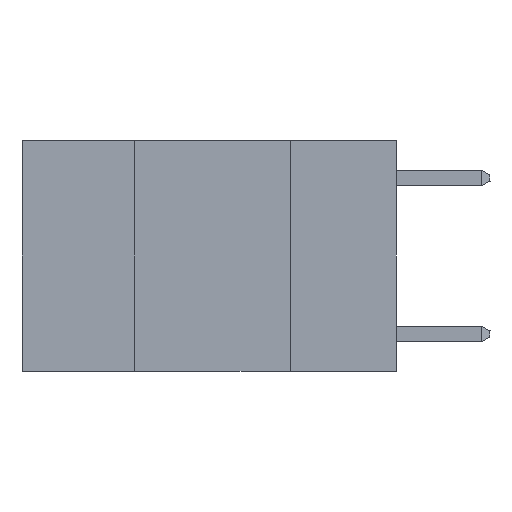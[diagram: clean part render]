
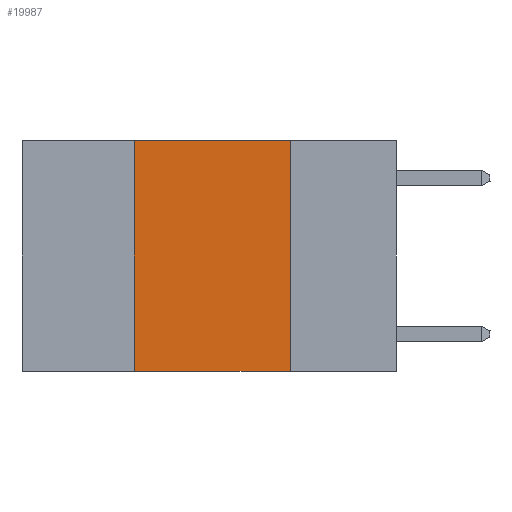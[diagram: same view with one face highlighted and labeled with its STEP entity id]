
A CAD part, left-side view. The second image highlights one B-rep face of the part: STEP entity #19987.
In plain terms, the highlighted planar face has unit normal (-1, 0, 0).
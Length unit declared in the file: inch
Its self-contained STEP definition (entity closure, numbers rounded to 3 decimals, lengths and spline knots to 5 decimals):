
#81 = ORIENTED_EDGE ( 'NONE', *, *, #4656, .F. ) ;
#88 = DIRECTION ( 'NONE',  ( 0., 0., -1. ) ) ;
#126 = CARTESIAN_POINT ( 'NONE',  ( 0., 0.42, -0.37 ) ) ;
#764 = VERTEX_POINT ( 'NONE', #18669 ) ;
#800 = CARTESIAN_POINT ( 'NONE',  ( 0., 0.6, 0. ) ) ;
#1020 = ORIENTED_EDGE ( 'NONE', *, *, #28578, .T. ) ;
#1370 = VECTOR ( 'NONE', #3851, 39.37008 ) ;
#1443 = ORIENTED_EDGE ( 'NONE', *, *, #11536, .F. ) ;
#1786 = DIRECTION ( 'NONE',  ( 0., -1., 0. ) ) ;
#3423 = VECTOR ( 'NONE', #21287, 39.37008 ) ;
#3851 = DIRECTION ( 'NONE',  ( 0., 0., 1. ) ) ;
#4656 = EDGE_CURVE ( 'NONE', #15846, #764, #14714, .T. ) ;
#6048 = VECTOR ( 'NONE', #1786, 39.37008 ) ;
#7140 = PLANE ( 'NONE',  #13299 ) ;
#7688 = LINE ( 'NONE', #22243, #1370 ) ;
#8535 = VECTOR ( 'NONE', #26235, 39.37008 ) ;
#8671 = VERTEX_POINT ( 'NONE', #22958 ) ;
#11536 = EDGE_CURVE ( 'NONE', #764, #8671, #21907, .T. ) ;
#13299 = AXIS2_PLACEMENT_3D ( 'NONE', #27609, #14152, #88 ) ;
#13566 = EDGE_LOOP ( 'NONE', ( #1443, #81, #16326, #1020 ) ) ;
#14152 = DIRECTION ( 'NONE',  ( 1., 0., 0. ) ) ;
#14714 = LINE ( 'NONE', #800, #8535 ) ;
#15846 = VERTEX_POINT ( 'NONE', #18773 ) ;
#16326 = ORIENTED_EDGE ( 'NONE', *, *, #21149, .F. ) ;
#16833 = FACE_OUTER_BOUND ( 'NONE', #13566, .T. ) ;
#18669 = CARTESIAN_POINT ( 'NONE',  ( 0., 0.17, 0. ) ) ;
#18773 = CARTESIAN_POINT ( 'NONE',  ( 0., 0.42, 0. ) ) ;
#18982 = CARTESIAN_POINT ( 'NONE',  ( 0., 0.17, 0. ) ) ;
#19987 = ADVANCED_FACE ( 'NONE', ( #16833 ), #7140, .F. ) ;
#21149 = EDGE_CURVE ( 'NONE', #28728, #15846, #7688, .T. ) ;
#21287 = DIRECTION ( 'NONE',  ( 0., 0., -1. ) ) ;
#21907 = LINE ( 'NONE', #18982, #3423 ) ;
#22243 = CARTESIAN_POINT ( 'NONE',  ( 0., 0.42, 0. ) ) ;
#22958 = CARTESIAN_POINT ( 'NONE',  ( 0., 0.17, -0.37 ) ) ;
#25003 = LINE ( 'NONE', #27071, #6048 ) ;
#26235 = DIRECTION ( 'NONE',  ( 0., -1., 0. ) ) ;
#27071 = CARTESIAN_POINT ( 'NONE',  ( 0., 0.6, -0.37 ) ) ;
#27609 = CARTESIAN_POINT ( 'NONE',  ( 0., 0.6, 0. ) ) ;
#28578 = EDGE_CURVE ( 'NONE', #28728, #8671, #25003, .T. ) ;
#28728 = VERTEX_POINT ( 'NONE', #126 ) ;
